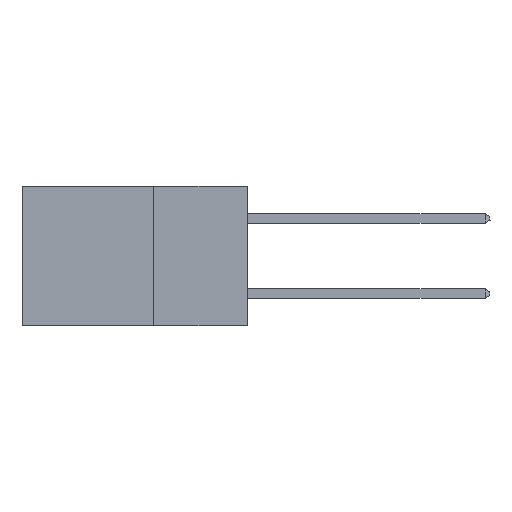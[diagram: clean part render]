
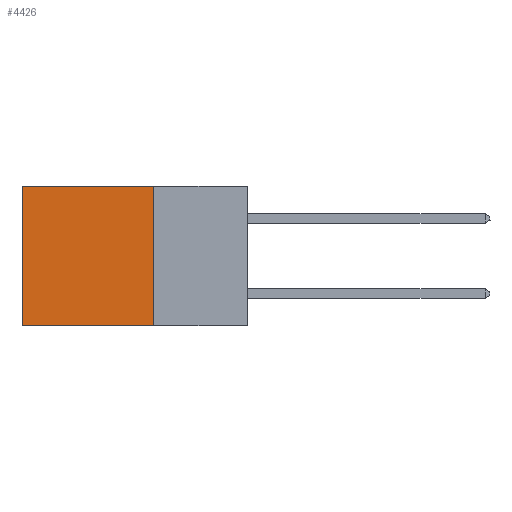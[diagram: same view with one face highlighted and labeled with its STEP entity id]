
A CAD part, left-side view. The second image highlights one B-rep face of the part: STEP entity #4426.
In plain terms, the highlighted planar face has unit normal (-1, 0, 0).
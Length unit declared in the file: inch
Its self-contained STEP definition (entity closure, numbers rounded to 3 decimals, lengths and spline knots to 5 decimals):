
#1212 = CARTESIAN_POINT ( 'NONE',  ( 0.2615, 0.25, -0.37 ) ) ;
#1402 = VERTEX_POINT ( 'NONE', #3643 ) ;
#1652 = EDGE_CURVE ( 'NONE', #1402, #12930, #9749, .T. ) ;
#1991 = DIRECTION ( 'NONE',  ( 0., 1., 0. ) ) ;
#2960 = ORIENTED_EDGE ( 'NONE', *, *, #1652, .F. ) ;
#2981 = DIRECTION ( 'NONE',  ( 0., 0., -1. ) ) ;
#3021 = DIRECTION ( 'NONE',  ( 0., 0., -1. ) ) ;
#3643 = CARTESIAN_POINT ( 'NONE',  ( 0.2615, 0.25, -0.37 ) ) ;
#4223 = DIRECTION ( 'NONE',  ( 0., 1., 0. ) ) ;
#4426 = ADVANCED_FACE ( 'NONE', ( #8402 ), #10060, .F. ) ;
#4877 = EDGE_CURVE ( 'NONE', #21239, #9481, #16617, .T. ) ;
#6568 = ORIENTED_EDGE ( 'NONE', *, *, #4877, .T. ) ;
#7285 = VECTOR ( 'NONE', #4223, 39.37008 ) ;
#8197 = ORIENTED_EDGE ( 'NONE', *, *, #11946, .T. ) ;
#8402 = FACE_OUTER_BOUND ( 'NONE', #22087, .T. ) ;
#8710 = CARTESIAN_POINT ( 'NONE',  ( 0.2615, 0.25, 0. ) ) ;
#9085 = LINE ( 'NONE', #20396, #17307 ) ;
#9371 = EDGE_CURVE ( 'NONE', #21239, #1402, #22488, .T. ) ;
#9481 = VERTEX_POINT ( 'NONE', #12167 ) ;
#9749 = LINE ( 'NONE', #12037, #17957 ) ;
#10060 = PLANE ( 'NONE',  #19458 ) ;
#11835 = CARTESIAN_POINT ( 'NONE',  ( 0.2615, 0.25, -0.37 ) ) ;
#11946 = EDGE_CURVE ( 'NONE', #9481, #12930, #9085, .T. ) ;
#12037 = CARTESIAN_POINT ( 'NONE',  ( 0.2615, 0.25, -0.37 ) ) ;
#12167 = CARTESIAN_POINT ( 'NONE',  ( 0.2615, 0.6, 0. ) ) ;
#12930 = VERTEX_POINT ( 'NONE', #15998 ) ;
#13594 = DIRECTION ( 'NONE',  ( 1., 0., 0. ) ) ;
#13725 = VECTOR ( 'NONE', #3021, 39.37008 ) ;
#15998 = CARTESIAN_POINT ( 'NONE',  ( 0.2615, 0.6, -0.37 ) ) ;
#16221 = ORIENTED_EDGE ( 'NONE', *, *, #9371, .F. ) ;
#16617 = LINE ( 'NONE', #19973, #7285 ) ;
#17307 = VECTOR ( 'NONE', #18716, 39.37008 ) ;
#17957 = VECTOR ( 'NONE', #1991, 39.37008 ) ;
#18716 = DIRECTION ( 'NONE',  ( 0., 0., -1. ) ) ;
#19458 = AXIS2_PLACEMENT_3D ( 'NONE', #11835, #13594, #2981 ) ;
#19973 = CARTESIAN_POINT ( 'NONE',  ( 0.2615, 0.25, 0. ) ) ;
#20396 = CARTESIAN_POINT ( 'NONE',  ( 0.2615, 0.6, -0.37 ) ) ;
#21239 = VERTEX_POINT ( 'NONE', #8710 ) ;
#22087 = EDGE_LOOP ( 'NONE', ( #8197, #2960, #16221, #6568 ) ) ;
#22488 = LINE ( 'NONE', #1212, #13725 ) ;
